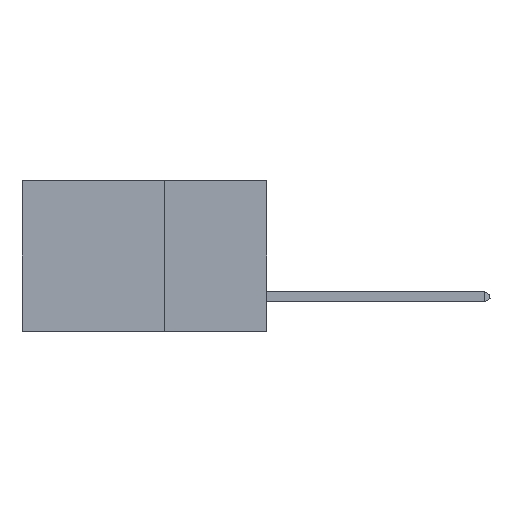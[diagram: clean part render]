
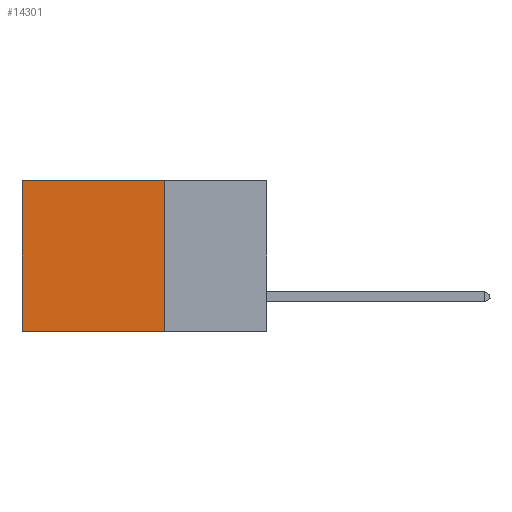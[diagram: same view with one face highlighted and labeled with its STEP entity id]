
A CAD part, left-side view. The second image highlights one B-rep face of the part: STEP entity #14301.
In plain terms, the highlighted planar face has unit normal (-1, 0, 0).
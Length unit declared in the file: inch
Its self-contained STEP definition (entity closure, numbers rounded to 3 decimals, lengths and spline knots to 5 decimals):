
#59 = LINE ( 'NONE', #24000, #15897 ) ;
#891 = CARTESIAN_POINT ( 'NONE',  ( 0.2875, 0.6, 0. ) ) ;
#1179 = CARTESIAN_POINT ( 'NONE',  ( 0.2875, 0.6, -0.37 ) ) ;
#1648 = CARTESIAN_POINT ( 'NONE',  ( 0.2875, 0.25, 0. ) ) ;
#2461 = VECTOR ( 'NONE', #13901, 39.37008 ) ;
#2891 = DIRECTION ( 'NONE',  ( 0., 0., -1. ) ) ;
#2929 = VERTEX_POINT ( 'NONE', #16593 ) ;
#3811 = ORIENTED_EDGE ( 'NONE', *, *, #6884, .T. ) ;
#4308 = EDGE_LOOP ( 'NONE', ( #3811, #11986, #18048, #12952 ) ) ;
#4428 = CARTESIAN_POINT ( 'NONE',  ( 0.2875, 0.25, -0.37 ) ) ;
#6006 = LINE ( 'NONE', #15408, #19874 ) ;
#6030 = EDGE_CURVE ( 'NONE', #7813, #6590, #16963, .T. ) ;
#6590 = VERTEX_POINT ( 'NONE', #1179 ) ;
#6884 = EDGE_CURVE ( 'NONE', #16783, #6590, #13343, .T. ) ;
#7119 = CARTESIAN_POINT ( 'NONE',  ( 0.2875, 0.6, 0. ) ) ;
#7813 = VERTEX_POINT ( 'NONE', #4428 ) ;
#7840 = CARTESIAN_POINT ( 'NONE',  ( 0.2875, 0.25, -0.37 ) ) ;
#7843 = DIRECTION ( 'NONE',  ( 0., 0., -1. ) ) ;
#8962 = AXIS2_PLACEMENT_3D ( 'NONE', #1648, #13906, #7843 ) ;
#11797 = DIRECTION ( 'NONE',  ( 0., 0., -1. ) ) ;
#11986 = ORIENTED_EDGE ( 'NONE', *, *, #6030, .F. ) ;
#12740 = EDGE_CURVE ( 'NONE', #2929, #7813, #6006, .T. ) ;
#12952 = ORIENTED_EDGE ( 'NONE', *, *, #22583, .T. ) ;
#13343 = LINE ( 'NONE', #7119, #15631 ) ;
#13901 = DIRECTION ( 'NONE',  ( 0., 1., 0. ) ) ;
#13906 = DIRECTION ( 'NONE',  ( 1., 0., 0. ) ) ;
#14301 = ADVANCED_FACE ( 'NONE', ( #23630 ), #22088, .F. ) ;
#15408 = CARTESIAN_POINT ( 'NONE',  ( 0.2875, 0.25, 0. ) ) ;
#15461 = DIRECTION ( 'NONE',  ( 0., 1., 0. ) ) ;
#15631 = VECTOR ( 'NONE', #11797, 39.37008 ) ;
#15897 = VECTOR ( 'NONE', #15461, 39.37008 ) ;
#16593 = CARTESIAN_POINT ( 'NONE',  ( 0.2875, 0.25, 0. ) ) ;
#16783 = VERTEX_POINT ( 'NONE', #891 ) ;
#16963 = LINE ( 'NONE', #7840, #2461 ) ;
#18048 = ORIENTED_EDGE ( 'NONE', *, *, #12740, .F. ) ;
#19874 = VECTOR ( 'NONE', #2891, 39.37008 ) ;
#22088 = PLANE ( 'NONE',  #8962 ) ;
#22583 = EDGE_CURVE ( 'NONE', #2929, #16783, #59, .T. ) ;
#23630 = FACE_OUTER_BOUND ( 'NONE', #4308, .T. ) ;
#24000 = CARTESIAN_POINT ( 'NONE',  ( 0.2875, 0.25, 0. ) ) ;
